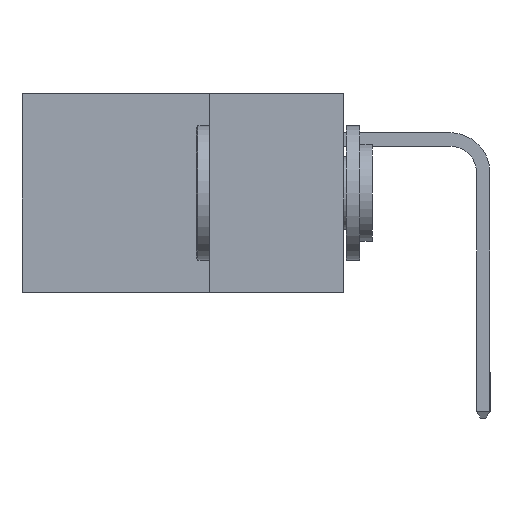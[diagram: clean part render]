
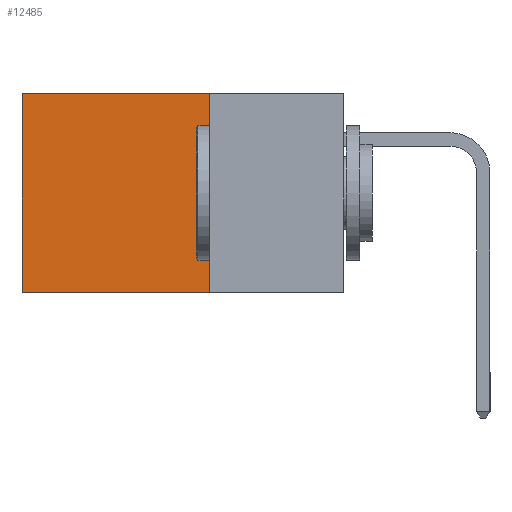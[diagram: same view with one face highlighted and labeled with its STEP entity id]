
A CAD part, left-side view. The second image highlights one B-rep face of the part: STEP entity #12485.
In plain terms, the highlighted planar face has unit normal (-1, 0, 0).
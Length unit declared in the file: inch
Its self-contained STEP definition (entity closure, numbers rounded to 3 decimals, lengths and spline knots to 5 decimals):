
#91 = DIRECTION ( 'NONE',  ( 0., 1., 0. ) ) ;
#837 = DIRECTION ( 'NONE',  ( 0., 0., -1. ) ) ;
#1588 = VERTEX_POINT ( 'NONE', #16850 ) ;
#3240 = CARTESIAN_POINT ( 'NONE',  ( 0.2615, 0.25, 0. ) ) ;
#3627 = VECTOR ( 'NONE', #19702, 39.37008 ) ;
#3705 = CARTESIAN_POINT ( 'NONE',  ( 0.2615, 0.25, -0.37 ) ) ;
#3784 = DIRECTION ( 'NONE',  ( 0., 0., -1. ) ) ;
#4447 = ORIENTED_EDGE ( 'NONE', *, *, #11173, .T. ) ;
#4592 = EDGE_CURVE ( 'NONE', #20792, #1588, #15811, .T. ) ;
#4952 = AXIS2_PLACEMENT_3D ( 'NONE', #6715, #13227, #16655 ) ;
#5514 = CARTESIAN_POINT ( 'NONE',  ( 0.2615, 0.6, -0.37 ) ) ;
#5535 = VERTEX_POINT ( 'NONE', #14235 ) ;
#5698 = CARTESIAN_POINT ( 'NONE',  ( 0.2615, 0.6, -0.37 ) ) ;
#5905 = ORIENTED_EDGE ( 'NONE', *, *, #13792, .T. ) ;
#5946 = VECTOR ( 'NONE', #3784, 39.37008 ) ;
#6715 = CARTESIAN_POINT ( 'NONE',  ( 0.2615, 0.25, -0.37 ) ) ;
#7489 = VECTOR ( 'NONE', #837, 39.37008 ) ;
#8322 = PLANE ( 'NONE',  #4952 ) ;
#8846 = CARTESIAN_POINT ( 'NONE',  ( 0.2615, 0.25, 0. ) ) ;
#9067 = VECTOR ( 'NONE', #91, 39.37008 ) ;
#9161 = EDGE_LOOP ( 'NONE', ( #4447, #13435, #21029, #5905 ) ) ;
#10502 = EDGE_CURVE ( 'NONE', #1588, #16239, #13217, .T. ) ;
#11173 = EDGE_CURVE ( 'NONE', #5535, #16239, #16727, .T. ) ;
#11661 = LINE ( 'NONE', #3240, #3627 ) ;
#12485 = ADVANCED_FACE ( 'NONE', ( #19675 ), #8322, .F. ) ;
#13217 = LINE ( 'NONE', #3705, #9067 ) ;
#13227 = DIRECTION ( 'NONE',  ( 1., 0., 0. ) ) ;
#13435 = ORIENTED_EDGE ( 'NONE', *, *, #10502, .F. ) ;
#13792 = EDGE_CURVE ( 'NONE', #20792, #5535, #11661, .T. ) ;
#14235 = CARTESIAN_POINT ( 'NONE',  ( 0.2615, 0.6, 0. ) ) ;
#15811 = LINE ( 'NONE', #20844, #7489 ) ;
#16239 = VERTEX_POINT ( 'NONE', #5514 ) ;
#16655 = DIRECTION ( 'NONE',  ( 0., 0., -1. ) ) ;
#16727 = LINE ( 'NONE', #5698, #5946 ) ;
#16850 = CARTESIAN_POINT ( 'NONE',  ( 0.2615, 0.25, -0.37 ) ) ;
#19675 = FACE_OUTER_BOUND ( 'NONE', #9161, .T. ) ;
#19702 = DIRECTION ( 'NONE',  ( 0., 1., 0. ) ) ;
#20792 = VERTEX_POINT ( 'NONE', #8846 ) ;
#20844 = CARTESIAN_POINT ( 'NONE',  ( 0.2615, 0.25, -0.37 ) ) ;
#21029 = ORIENTED_EDGE ( 'NONE', *, *, #4592, .F. ) ;
